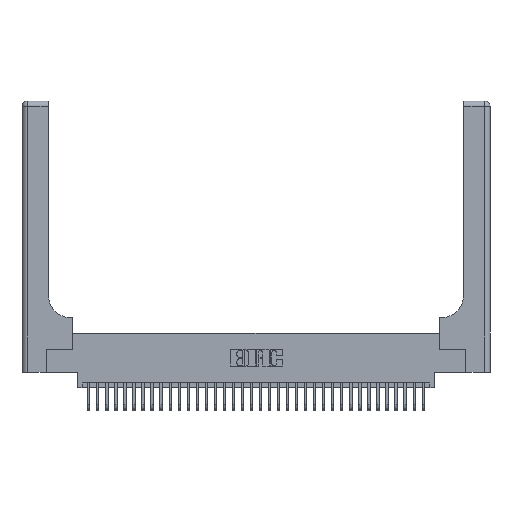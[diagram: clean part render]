
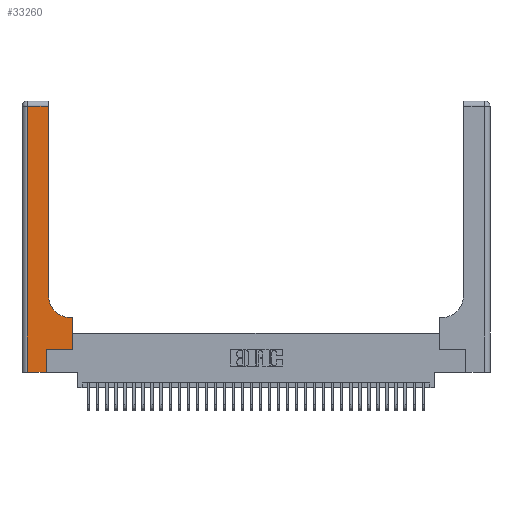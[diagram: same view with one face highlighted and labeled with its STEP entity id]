
A CAD part, top view. The second image highlights one B-rep face of the part: STEP entity #33260.
In plain terms, the highlighted planar face has unit normal (0, 0, 1).
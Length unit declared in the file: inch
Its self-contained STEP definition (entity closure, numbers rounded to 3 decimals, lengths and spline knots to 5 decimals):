
#113 = LINE ( 'NONE', #18579, #26814 ) ;
#512 = DIRECTION ( 'NONE',  ( -1., 0., 0. ) ) ;
#827 = LINE ( 'NONE', #18314, #28356 ) ;
#1600 = DIRECTION ( 'NONE',  ( 1., 0., 0. ) ) ;
#2079 = CARTESIAN_POINT ( 'NONE',  ( 0., 0., 0.37 ) ) ;
#2511 = LINE ( 'NONE', #18245, #30020 ) ;
#2557 = ORIENTED_EDGE ( 'NONE', *, *, #33868, .T. ) ;
#3451 = EDGE_CURVE ( 'NONE', #11723, #4796, #827, .T. ) ;
#4581 = CARTESIAN_POINT ( 'NONE',  ( 0.269, 0., 0.37 ) ) ;
#4600 = ORIENTED_EDGE ( 'NONE', *, *, #20151, .T. ) ;
#4796 = VERTEX_POINT ( 'NONE', #16371 ) ;
#4924 = VECTOR ( 'NONE', #13420, 39.37008 ) ;
#5200 = VECTOR ( 'NONE', #18896, 39.37008 ) ;
#6567 = LINE ( 'NONE', #16349, #27011 ) ;
#7575 = EDGE_CURVE ( 'NONE', #9254, #9249, #13145, .T. ) ;
#8066 = CARTESIAN_POINT ( 'NONE',  ( 0.5585, 0.25, 0.37 ) ) ;
#9249 = VERTEX_POINT ( 'NONE', #10114 ) ;
#9254 = VERTEX_POINT ( 'NONE', #12770 ) ;
#9772 = CARTESIAN_POINT ( 'NONE',  ( 0.5585, 0.6, 0.37 ) ) ;
#10114 = CARTESIAN_POINT ( 'NONE',  ( 0.2915, 0.85, 0.37 ) ) ;
#10957 = CARTESIAN_POINT ( 'NONE',  ( 0., 3., 0.37 ) ) ;
#11047 = VERTEX_POINT ( 'NONE', #22622 ) ;
#11392 = VECTOR ( 'NONE', #12993, 39.37008 ) ;
#11723 = VERTEX_POINT ( 'NONE', #4581 ) ;
#12192 = CARTESIAN_POINT ( 'NONE',  ( 0.06, 2.94, 0.37 ) ) ;
#12770 = CARTESIAN_POINT ( 'NONE',  ( 0.5415, 0.6, 0.37 ) ) ;
#12993 = DIRECTION ( 'NONE',  ( 1., 0., 0. ) ) ;
#13145 = CIRCLE ( 'NONE', #28498, 0.25 ) ;
#13420 = DIRECTION ( 'NONE',  ( 0., 1., 0. ) ) ;
#13544 = AXIS2_PLACEMENT_3D ( 'NONE', #10957, #29572, #13604 ) ;
#13604 = DIRECTION ( 'NONE',  ( -1., 0., 0. ) ) ;
#13687 = EDGE_CURVE ( 'NONE', #4796, #11047, #24728, .T. ) ;
#13782 = VERTEX_POINT ( 'NONE', #12192 ) ;
#14400 = ORIENTED_EDGE ( 'NONE', *, *, #13687, .T. ) ;
#15473 = CARTESIAN_POINT ( 'NONE',  ( 0.06, 0., 0.37 ) ) ;
#15627 = DIRECTION ( 'NONE',  ( 0., 1., 0. ) ) ;
#15665 = DIRECTION ( 'NONE',  ( 0., -1., 0. ) ) ;
#15733 = EDGE_CURVE ( 'NONE', #9249, #32796, #26219, .T. ) ;
#16095 = CARTESIAN_POINT ( 'NONE',  ( 0.2915, 3., 0.37 ) ) ;
#16349 = CARTESIAN_POINT ( 'NONE',  ( 0., 2.94, 0.37 ) ) ;
#16371 = CARTESIAN_POINT ( 'NONE',  ( 0.269, 0.25, 0.37 ) ) ;
#17380 = ORIENTED_EDGE ( 'NONE', *, *, #3451, .T. ) ;
#17556 = DIRECTION ( 'NONE',  ( 0., 0., -1. ) ) ;
#18024 = FACE_OUTER_BOUND ( 'NONE', #29818, .T. ) ;
#18245 = CARTESIAN_POINT ( 'NONE',  ( 0.06, 3., 0.37 ) ) ;
#18314 = CARTESIAN_POINT ( 'NONE',  ( 0.269, 0., 0.37 ) ) ;
#18560 = LINE ( 'NONE', #8066, #5200 ) ;
#18579 = CARTESIAN_POINT ( 'NONE',  ( 0.2915, 0.6, 0.37 ) ) ;
#18836 = ORIENTED_EDGE ( 'NONE', *, *, #7575, .T. ) ;
#18896 = DIRECTION ( 'NONE',  ( 0., 1., 0. ) ) ;
#18975 = ORIENTED_EDGE ( 'NONE', *, *, #26227, .T. ) ;
#19170 = VERTEX_POINT ( 'NONE', #9772 ) ;
#20151 = EDGE_CURVE ( 'NONE', #11047, #19170, #18560, .T. ) ;
#20599 = VERTEX_POINT ( 'NONE', #15473 ) ;
#21281 = DIRECTION ( 'NONE',  ( -1., 0., 0. ) ) ;
#22622 = CARTESIAN_POINT ( 'NONE',  ( 0.5585, 0.25, 0.37 ) ) ;
#23613 = EDGE_CURVE ( 'NONE', #13782, #20599, #2511, .T. ) ;
#24728 = LINE ( 'NONE', #31610, #11392 ) ;
#25248 = EDGE_CURVE ( 'NONE', #32796, #13782, #6567, .T. ) ;
#25820 = ORIENTED_EDGE ( 'NONE', *, *, #23613, .T. ) ;
#26209 = DIRECTION ( 'NONE',  ( 1., 0., 0. ) ) ;
#26219 = LINE ( 'NONE', #16095, #4924 ) ;
#26227 = EDGE_CURVE ( 'NONE', #20599, #11723, #26573, .T. ) ;
#26573 = LINE ( 'NONE', #2079, #33640 ) ;
#26814 = VECTOR ( 'NONE', #21281, 39.37008 ) ;
#27011 = VECTOR ( 'NONE', #512, 39.37008 ) ;
#28298 = CARTESIAN_POINT ( 'NONE',  ( 0.2915, 2.94, 0.37 ) ) ;
#28356 = VECTOR ( 'NONE', #15627, 39.37008 ) ;
#28498 = AXIS2_PLACEMENT_3D ( 'NONE', #33517, #17556, #1600 ) ;
#29572 = DIRECTION ( 'NONE',  ( 0., 0., -1. ) ) ;
#29818 = EDGE_LOOP ( 'NONE', ( #30448, #32607, #25820, #18975, #17380, #14400, #4600, #2557, #18836 ) ) ;
#30020 = VECTOR ( 'NONE', #15665, 39.37008 ) ;
#30448 = ORIENTED_EDGE ( 'NONE', *, *, #15733, .T. ) ;
#31610 = CARTESIAN_POINT ( 'NONE',  ( 0.269, 0.25, 0.37 ) ) ;
#32122 = PLANE ( 'NONE',  #13544 ) ;
#32607 = ORIENTED_EDGE ( 'NONE', *, *, #25248, .T. ) ;
#32796 = VERTEX_POINT ( 'NONE', #28298 ) ;
#33260 = ADVANCED_FACE ( 'NONE', ( #18024 ), #32122, .F. ) ;
#33517 = CARTESIAN_POINT ( 'NONE',  ( 0.5415, 0.85, 0.37 ) ) ;
#33640 = VECTOR ( 'NONE', #26209, 39.37008 ) ;
#33868 = EDGE_CURVE ( 'NONE', #19170, #9254, #113, .T. ) ;
